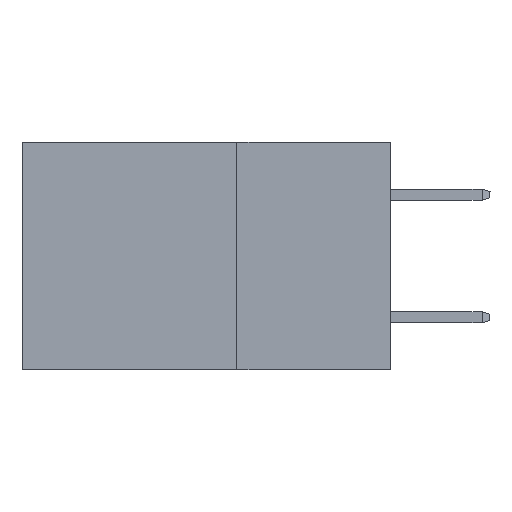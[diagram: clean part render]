
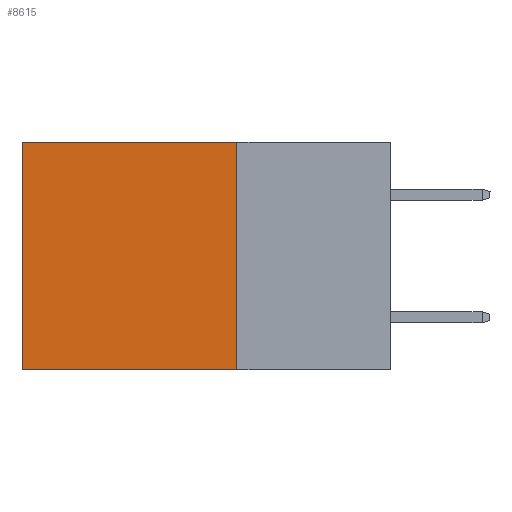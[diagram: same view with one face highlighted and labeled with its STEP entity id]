
A CAD part, left-side view. The second image highlights one B-rep face of the part: STEP entity #8615.
In plain terms, the highlighted planar face has unit normal (-1, 0, 0).
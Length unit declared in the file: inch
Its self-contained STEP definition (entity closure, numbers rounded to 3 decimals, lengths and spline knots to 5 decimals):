
#537 = LINE ( 'NONE', #3623, #5345 ) ;
#791 = EDGE_CURVE ( 'NONE', #12019, #10357, #9399, .T. ) ;
#941 = CARTESIAN_POINT ( 'NONE',  ( 0.2875, 0.25, 0. ) ) ;
#1234 = VECTOR ( 'NONE', #3714, 39.37008 ) ;
#1930 = FACE_OUTER_BOUND ( 'NONE', #11604, .T. ) ;
#2193 = CARTESIAN_POINT ( 'NONE',  ( 0.2875, 0.6, 0. ) ) ;
#3590 = CARTESIAN_POINT ( 'NONE',  ( 0.2875, 0.25, -0.37 ) ) ;
#3595 = ORIENTED_EDGE ( 'NONE', *, *, #12028, .T. ) ;
#3623 = CARTESIAN_POINT ( 'NONE',  ( 0.2875, 0.6, 0. ) ) ;
#3714 = DIRECTION ( 'NONE',  ( 0., 1., 0. ) ) ;
#3748 = AXIS2_PLACEMENT_3D ( 'NONE', #4156, #10791, #5137 ) ;
#3779 = ORIENTED_EDGE ( 'NONE', *, *, #3838, .T. ) ;
#3838 = EDGE_CURVE ( 'NONE', #10499, #10357, #537, .T. ) ;
#4156 = CARTESIAN_POINT ( 'NONE',  ( 0.2875, 0.25, 0. ) ) ;
#4473 = ORIENTED_EDGE ( 'NONE', *, *, #4875, .F. ) ;
#4875 = EDGE_CURVE ( 'NONE', #5056, #12019, #9209, .T. ) ;
#5056 = VERTEX_POINT ( 'NONE', #941 ) ;
#5137 = DIRECTION ( 'NONE',  ( 0., 0., -1. ) ) ;
#5345 = VECTOR ( 'NONE', #6278, 39.37008 ) ;
#5718 = DIRECTION ( 'NONE',  ( 0., 0., -1. ) ) ;
#6057 = ORIENTED_EDGE ( 'NONE', *, *, #791, .F. ) ;
#6278 = DIRECTION ( 'NONE',  ( 0., 0., -1. ) ) ;
#7006 = PLANE ( 'NONE',  #3748 ) ;
#7796 = CARTESIAN_POINT ( 'NONE',  ( 0.2875, 0.6, -0.37 ) ) ;
#7858 = CARTESIAN_POINT ( 'NONE',  ( 0.2875, 0.25, 0. ) ) ;
#8615 = ADVANCED_FACE ( 'NONE', ( #1930 ), #7006, .F. ) ;
#8626 = DIRECTION ( 'NONE',  ( 0., 1., 0. ) ) ;
#8896 = LINE ( 'NONE', #11280, #1234 ) ;
#9209 = LINE ( 'NONE', #7858, #11356 ) ;
#9399 = LINE ( 'NONE', #3590, #11537 ) ;
#10357 = VERTEX_POINT ( 'NONE', #7796 ) ;
#10499 = VERTEX_POINT ( 'NONE', #2193 ) ;
#10791 = DIRECTION ( 'NONE',  ( 1., 0., 0. ) ) ;
#11238 = CARTESIAN_POINT ( 'NONE',  ( 0.2875, 0.25, -0.37 ) ) ;
#11280 = CARTESIAN_POINT ( 'NONE',  ( 0.2875, 0.25, 0. ) ) ;
#11356 = VECTOR ( 'NONE', #5718, 39.37008 ) ;
#11537 = VECTOR ( 'NONE', #8626, 39.37008 ) ;
#11604 = EDGE_LOOP ( 'NONE', ( #3779, #6057, #4473, #3595 ) ) ;
#12019 = VERTEX_POINT ( 'NONE', #11238 ) ;
#12028 = EDGE_CURVE ( 'NONE', #5056, #10499, #8896, .T. ) ;
